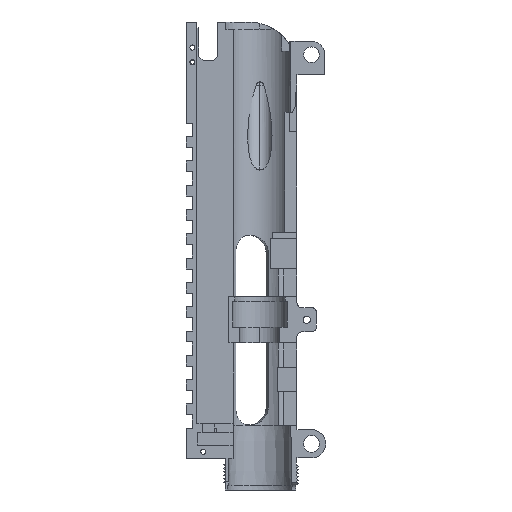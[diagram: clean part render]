
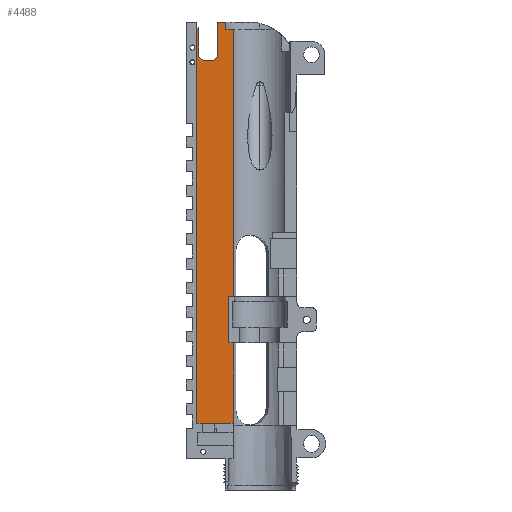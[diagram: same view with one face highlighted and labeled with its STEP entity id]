
A CAD part, left-side view. The second image highlights one B-rep face of the part: STEP entity #4488.
In plain terms, the highlighted planar face has unit normal (-1, 0, 0).
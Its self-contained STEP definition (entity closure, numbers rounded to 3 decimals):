
#25 = LINE ( 'NONE', #7538, #6331 ) ;
#178 = CARTESIAN_POINT ( 'NONE',  ( 6.4, 0., -3. ) ) ;
#185 = CARTESIAN_POINT ( 'NONE',  ( 6.4, 19.25, -16. ) ) ;
#226 = CARTESIAN_POINT ( 'NONE',  ( 6.4, 25.95, -165. ) ) ;
#233 = CARTESIAN_POINT ( 'NONE',  ( 6.4, 12.75, -132. ) ) ;
#316 = VERTEX_POINT ( 'NONE', #7565 ) ;
#507 = VERTEX_POINT ( 'NONE', #10727 ) ;
#548 = EDGE_CURVE ( 'NONE', #12833, #316, #9189, .T. ) ;
#609 = ORIENTED_EDGE ( 'NONE', *, *, #9976, .F. ) ;
#680 = LINE ( 'NONE', #10141, #13094 ) ;
#819 = VERTEX_POINT ( 'NONE', #13496 ) ;
#891 = ORIENTED_EDGE ( 'NONE', *, *, #12820, .F. ) ;
#1052 = DIRECTION ( 'NONE',  ( 0., 0., -1. ) ) ;
#1133 = CARTESIAN_POINT ( 'NONE',  ( 6.4, 11.027, -165. ) ) ;
#1232 = DIRECTION ( 'NONE',  ( 0., -0.707, -0.707 ) ) ;
#1349 = EDGE_CURVE ( 'NONE', #13795, #7602, #9426, .T. ) ;
#1388 = EDGE_CURVE ( 'NONE', #12833, #13795, #2248, .T. ) ;
#1617 = EDGE_CURVE ( 'NONE', #819, #10266, #13295, .T. ) ;
#1815 = ORIENTED_EDGE ( 'NONE', *, *, #5214, .F. ) ;
#1858 = CARTESIAN_POINT ( 'NONE',  ( 6.4, 23.25, -16. ) ) ;
#1873 = CARTESIAN_POINT ( 'NONE',  ( 6.4, 11.027, -3. ) ) ;
#1915 = ORIENTED_EDGE ( 'NONE', *, *, #1349, .F. ) ;
#2065 = DIRECTION ( 'NONE',  ( 0., 0., 1. ) ) ;
#2248 = LINE ( 'NONE', #7512, #6183 ) ;
#2369 = DIRECTION ( 'NONE',  ( 0., 1., 0. ) ) ;
#2643 = EDGE_CURVE ( 'NONE', #8287, #316, #7347, .T. ) ;
#2796 = ORIENTED_EDGE ( 'NONE', *, *, #9518, .F. ) ;
#2877 = LINE ( 'NONE', #10103, #4240 ) ;
#2879 = VERTEX_POINT ( 'NONE', #1873 ) ;
#3247 = VERTEX_POINT ( 'NONE', #185 ) ;
#3251 = DIRECTION ( 'NONE',  ( 0., 1., 0. ) ) ;
#3332 = DIRECTION ( 'NONE',  ( 0., -1., 0. ) ) ;
#3361 = CARTESIAN_POINT ( 'NONE',  ( 6.4, 25.25, -14. ) ) ;
#3365 = EDGE_CURVE ( 'NONE', #10266, #3247, #680, .T. ) ;
#3373 = CARTESIAN_POINT ( 'NONE',  ( 6.4, -27.051, -2.434 ) ) ;
#3474 = CARTESIAN_POINT ( 'NONE',  ( 6.4, 12.75, -132. ) ) ;
#3514 = DIRECTION ( 'NONE',  ( 0., -1., 0. ) ) ;
#3730 = VECTOR ( 'NONE', #3514, 1000. ) ;
#3786 = ORIENTED_EDGE ( 'NONE', *, *, #2643, .F. ) ;
#3820 = LINE ( 'NONE', #3373, #12335 ) ;
#3930 = VECTOR ( 'NONE', #1232, 1000. ) ;
#3937 = CARTESIAN_POINT ( 'NONE',  ( 6.4, 12.75, -132. ) ) ;
#4014 = ORIENTED_EDGE ( 'NONE', *, *, #9788, .T. ) ;
#4174 = CARTESIAN_POINT ( 'NONE',  ( 6.4, 11.027, 0. ) ) ;
#4240 = VECTOR ( 'NONE', #5624, 1000. ) ;
#4386 = LINE ( 'NONE', #178, #12385 ) ;
#4488 = ADVANCED_FACE ( 'NONE', ( #4539 ), #12266, .F. ) ;
#4537 = EDGE_CURVE ( 'NONE', #2879, #8584, #4386, .T. ) ;
#4539 = FACE_OUTER_BOUND ( 'NONE', #10803, .T. ) ;
#4584 = ORIENTED_EDGE ( 'NONE', *, *, #1617, .F. ) ;
#4837 = ORIENTED_EDGE ( 'NONE', *, *, #6257, .T. ) ;
#4938 = CARTESIAN_POINT ( 'NONE',  ( 6.4, 19.25, -16. ) ) ;
#5052 = VERTEX_POINT ( 'NONE', #7927 ) ;
#5147 = VECTOR ( 'NONE', #2065, 1000. ) ;
#5214 = EDGE_CURVE ( 'NONE', #3247, #10359, #13108, .T. ) ;
#5255 = VECTOR ( 'NONE', #11535, 1000. ) ;
#5333 = DIRECTION ( 'NONE',  ( 0., 0., 1. ) ) ;
#5624 = DIRECTION ( 'NONE',  ( 0., 0., 1. ) ) ;
#5637 = ORIENTED_EDGE ( 'NONE', *, *, #6489, .T. ) ;
#5966 = VECTOR ( 'NONE', #9077, 1000. ) ;
#6000 = DIRECTION ( 'NONE',  ( 0., -1., 0. ) ) ;
#6014 = LINE ( 'NONE', #12584, #14024 ) ;
#6103 = CARTESIAN_POINT ( 'NONE',  ( 6.4, 13.952, -3. ) ) ;
#6183 = VECTOR ( 'NONE', #6456, 1000. ) ;
#6257 = EDGE_CURVE ( 'NONE', #10944, #2879, #2877, .T. ) ;
#6275 = LINE ( 'NONE', #3937, #5255 ) ;
#6331 = VECTOR ( 'NONE', #9673, 1000. ) ;
#6430 = VERTEX_POINT ( 'NONE', #9200 ) ;
#6456 = DIRECTION ( 'NONE',  ( 0., 1., 0. ) ) ;
#6489 = EDGE_CURVE ( 'NONE', #8287, #8974, #6275, .T. ) ;
#6761 = EDGE_CURVE ( 'NONE', #5052, #819, #13597, .T. ) ;
#6810 = ORIENTED_EDGE ( 'NONE', *, *, #6761, .F. ) ;
#6971 = DIRECTION ( 'NONE',  ( 0., 1., 0. ) ) ;
#7054 = CARTESIAN_POINT ( 'NONE',  ( 6.4, 12.75, -113. ) ) ;
#7347 = LINE ( 'NONE', #3474, #3730 ) ;
#7512 = CARTESIAN_POINT ( 'NONE',  ( 6.4, 25.95, -165. ) ) ;
#7538 = CARTESIAN_POINT ( 'NONE',  ( 6.4, 17.25, -14. ) ) ;
#7565 = CARTESIAN_POINT ( 'NONE',  ( 6.4, 11.027, -132. ) ) ;
#7602 = VERTEX_POINT ( 'NONE', #10758 ) ;
#7927 = CARTESIAN_POINT ( 'NONE',  ( 6.4, 25.25, -2.434 ) ) ;
#8098 = VECTOR ( 'NONE', #3251, 1000. ) ;
#8287 = VERTEX_POINT ( 'NONE', #233 ) ;
#8457 = LINE ( 'NONE', #13294, #9659 ) ;
#8584 = VERTEX_POINT ( 'NONE', #6103 ) ;
#8607 = ORIENTED_EDGE ( 'NONE', *, *, #1388, .F. ) ;
#8974 = VERTEX_POINT ( 'NONE', #7054 ) ;
#9077 = DIRECTION ( 'NONE',  ( 0., -0.707, 0.707 ) ) ;
#9129 = LINE ( 'NONE', #10851, #8098 ) ;
#9189 = LINE ( 'NONE', #4174, #12239 ) ;
#9200 = CARTESIAN_POINT ( 'NONE',  ( 6.4, 17.25, 0. ) ) ;
#9332 = ORIENTED_EDGE ( 'NONE', *, *, #548, .T. ) ;
#9402 = CARTESIAN_POINT ( 'NONE',  ( 6.4, 11.027, -113. ) ) ;
#9426 = LINE ( 'NONE', #10759, #5147 ) ;
#9518 = EDGE_CURVE ( 'NONE', #507, #8584, #8457, .T. ) ;
#9659 = VECTOR ( 'NONE', #12342, 1000. ) ;
#9673 = DIRECTION ( 'NONE',  ( 0., 0., 1. ) ) ;
#9733 = CARTESIAN_POINT ( 'NONE',  ( 6.4, 17.25, -14. ) ) ;
#9788 = EDGE_CURVE ( 'NONE', #507, #6430, #9129, .T. ) ;
#9960 = ORIENTED_EDGE ( 'NONE', *, *, #12029, .F. ) ;
#9976 = EDGE_CURVE ( 'NONE', #7602, #5052, #3820, .T. ) ;
#10091 = AXIS2_PLACEMENT_3D ( 'NONE', #226, #11050, #2369 ) ;
#10103 = CARTESIAN_POINT ( 'NONE',  ( 6.4, 11.027, 0. ) ) ;
#10141 = CARTESIAN_POINT ( 'NONE',  ( 6.4, 23.25, -16. ) ) ;
#10266 = VERTEX_POINT ( 'NONE', #1858 ) ;
#10359 = VERTEX_POINT ( 'NONE', #9733 ) ;
#10603 = ORIENTED_EDGE ( 'NONE', *, *, #4537, .T. ) ;
#10727 = CARTESIAN_POINT ( 'NONE',  ( 6.4, 13.952, 0. ) ) ;
#10728 = VECTOR ( 'NONE', #1052, 1000. ) ;
#10758 = CARTESIAN_POINT ( 'NONE',  ( 6.4, 25.95, -2.434 ) ) ;
#10759 = CARTESIAN_POINT ( 'NONE',  ( 6.4, 25.95, -165. ) ) ;
#10803 = EDGE_LOOP ( 'NONE', ( #9960, #4837, #10603, #2796, #4014, #891, #1815, #13943, #4584, #6810, #609, #1915, #8607, #9332, #3786, #5637 ) ) ;
#10851 = CARTESIAN_POINT ( 'NONE',  ( 6.4, 25.95, 0. ) ) ;
#10944 = VERTEX_POINT ( 'NONE', #9402 ) ;
#11050 = DIRECTION ( 'NONE',  ( 1., 0., 0. ) ) ;
#11535 = DIRECTION ( 'NONE',  ( 0., 0., 1. ) ) ;
#12029 = EDGE_CURVE ( 'NONE', #10944, #8974, #6014, .T. ) ;
#12239 = VECTOR ( 'NONE', #5333, 1000. ) ;
#12266 = PLANE ( 'NONE',  #10091 ) ;
#12335 = VECTOR ( 'NONE', #3332, 1000. ) ;
#12342 = DIRECTION ( 'NONE',  ( 0., 0., -1. ) ) ;
#12385 = VECTOR ( 'NONE', #13349, 1000. ) ;
#12584 = CARTESIAN_POINT ( 'NONE',  ( 6.4, 11.027, -113. ) ) ;
#12820 = EDGE_CURVE ( 'NONE', #10359, #6430, #25, .T. ) ;
#12833 = VERTEX_POINT ( 'NONE', #1133 ) ;
#12938 = CARTESIAN_POINT ( 'NONE',  ( 6.4, 25.25, 0. ) ) ;
#13094 = VECTOR ( 'NONE', #6000, 1000. ) ;
#13108 = LINE ( 'NONE', #4938, #5966 ) ;
#13294 = CARTESIAN_POINT ( 'NONE',  ( 6.4, 13.952, -3. ) ) ;
#13295 = LINE ( 'NONE', #3361, #3930 ) ;
#13349 = DIRECTION ( 'NONE',  ( 0., 1., 0. ) ) ;
#13384 = CARTESIAN_POINT ( 'NONE',  ( 6.4, 25.95, -165. ) ) ;
#13496 = CARTESIAN_POINT ( 'NONE',  ( 6.4, 25.25, -14. ) ) ;
#13597 = LINE ( 'NONE', #12938, #10728 ) ;
#13795 = VERTEX_POINT ( 'NONE', #13384 ) ;
#13943 = ORIENTED_EDGE ( 'NONE', *, *, #3365, .F. ) ;
#14024 = VECTOR ( 'NONE', #6971, 1000. ) ;
